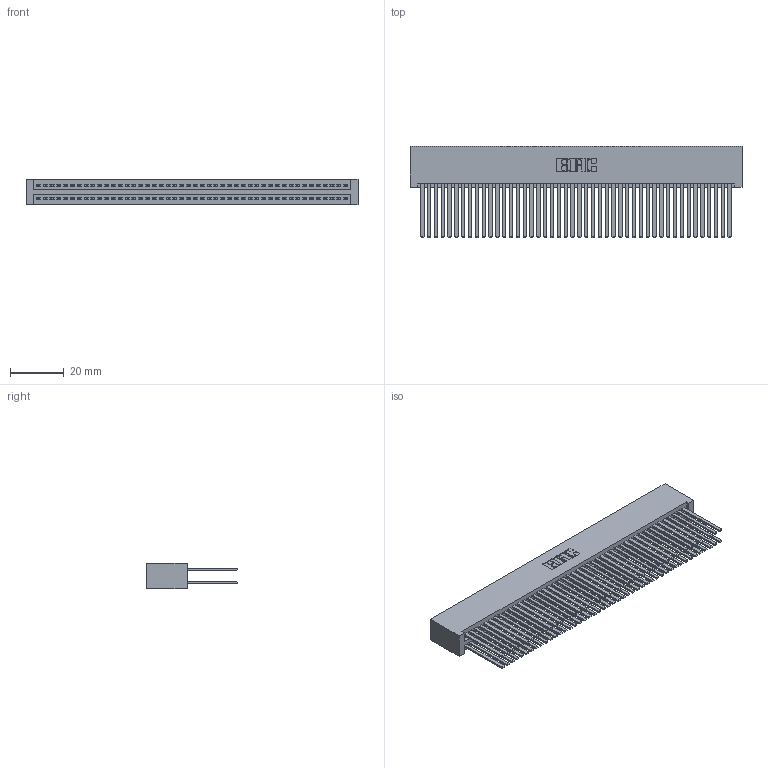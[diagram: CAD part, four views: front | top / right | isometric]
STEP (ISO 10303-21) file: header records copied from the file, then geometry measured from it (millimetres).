
FILE_DESCRIPTION (( 'STEP AP203' ), '1' );
FILE_NAME ('345-092-544-201.STEP', '2019-11-01T20:07:12', ( '' ), ( '' ), 'SwSTEP 2.0', 'SolidWorks 2016', '' );
FILE_SCHEMA (( 'CONFIG_CONTROL_DESIGN' ));
Length unit declared in the file: inch
Products named in the file (3): 345-092-544-201; 345-292-001_345-293-144; 345 Part_No Mounting Lugs
Assembly tree (93 placements, depth 2):
  345-092-544-201
    345 Part_No Mounting Lugs
    345-292-001_345-293-144  x92
Bounding box: 123.44 x 33.96 x 9.4 mm (x, y, z)
Volume: 13934.2 mm3; surface area: 24757.7 mm2
Topology: 93 solids, 93 shells, 4166 faces, 12369 edges, 8122 vertices
Faces by surface type: plane 2744, cylinder 1422
Entity records: 35093 total; most frequent: CARTESIAN_POINT 5876, ORIENTED_EDGE 5810, DIRECTION 5169, EDGE_CURVE 2905, VECTOR 2601, LINE 2601, VERTEX_POINT 1934, AXIS2_PLACEMENT_3D 1284
